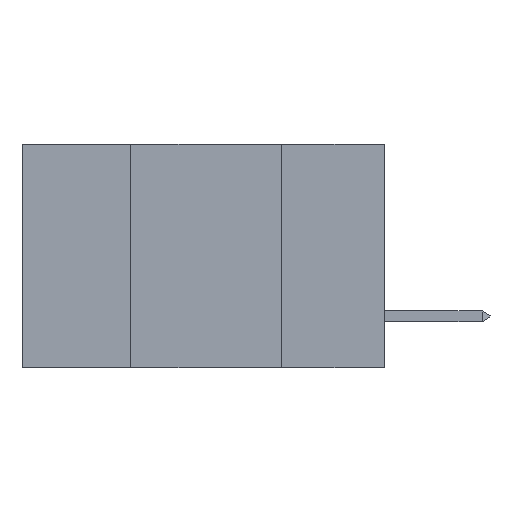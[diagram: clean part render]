
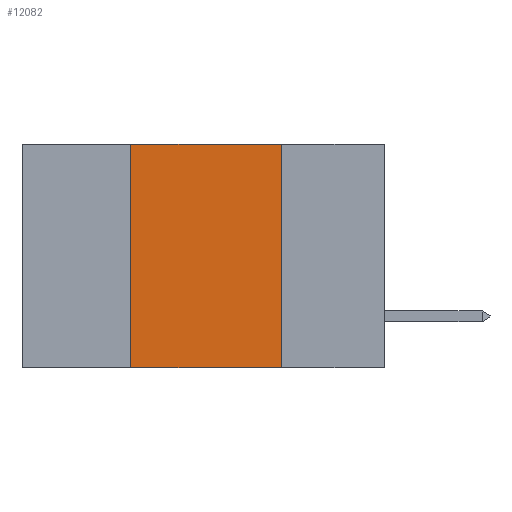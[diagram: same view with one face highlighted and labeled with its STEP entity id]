
A CAD part, left-side view. The second image highlights one B-rep face of the part: STEP entity #12082.
In plain terms, the highlighted planar face has unit normal (-1, 0, 0).
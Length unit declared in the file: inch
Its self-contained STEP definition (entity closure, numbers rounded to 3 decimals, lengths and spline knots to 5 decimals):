
#200 = VECTOR ( 'NONE', #7000, 39.37008 ) ;
#352 = LINE ( 'NONE', #3620, #3742 ) ;
#527 = ORIENTED_EDGE ( 'NONE', *, *, #12980, .T. ) ;
#578 = DIRECTION ( 'NONE',  ( 0., -1., 0. ) ) ;
#1085 = LINE ( 'NONE', #6597, #13701 ) ;
#1118 = CARTESIAN_POINT ( 'NONE',  ( 0., 0.42, 0. ) ) ;
#1951 = EDGE_CURVE ( 'NONE', #12165, #3316, #4775, .T. ) ;
#3173 = DIRECTION ( 'NONE',  ( 1., 0., 0. ) ) ;
#3300 = AXIS2_PLACEMENT_3D ( 'NONE', #7653, #3173, #4312 ) ;
#3316 = VERTEX_POINT ( 'NONE', #6538 ) ;
#3485 = DIRECTION ( 'NONE',  ( 0., -1., 0. ) ) ;
#3620 = CARTESIAN_POINT ( 'NONE',  ( 0., 0.6, -0.37 ) ) ;
#3742 = VECTOR ( 'NONE', #3485, 39.37008 ) ;
#4279 = EDGE_CURVE ( 'NONE', #8274, #12165, #8082, .T. ) ;
#4312 = DIRECTION ( 'NONE',  ( 0., 0., -1. ) ) ;
#4775 = LINE ( 'NONE', #7180, #8708 ) ;
#5139 = ORIENTED_EDGE ( 'NONE', *, *, #4279, .F. ) ;
#6538 = CARTESIAN_POINT ( 'NONE',  ( 0., 0.17, 0. ) ) ;
#6597 = CARTESIAN_POINT ( 'NONE',  ( 0., 0.17, 0. ) ) ;
#6686 = ORIENTED_EDGE ( 'NONE', *, *, #1951, .F. ) ;
#6718 = CARTESIAN_POINT ( 'NONE',  ( 0., 0.42, -0.37 ) ) ;
#7000 = DIRECTION ( 'NONE',  ( 0., 0., 1. ) ) ;
#7180 = CARTESIAN_POINT ( 'NONE',  ( 0., 0.6, 0. ) ) ;
#7653 = CARTESIAN_POINT ( 'NONE',  ( 0., 0.6, 0. ) ) ;
#8082 = LINE ( 'NONE', #1118, #200 ) ;
#8274 = VERTEX_POINT ( 'NONE', #6718 ) ;
#8708 = VECTOR ( 'NONE', #578, 39.37008 ) ;
#8733 = PLANE ( 'NONE',  #3300 ) ;
#10861 = VERTEX_POINT ( 'NONE', #12365 ) ;
#11112 = DIRECTION ( 'NONE',  ( 0., 0., -1. ) ) ;
#11236 = EDGE_CURVE ( 'NONE', #3316, #10861, #1085, .T. ) ;
#11942 = EDGE_LOOP ( 'NONE', ( #14010, #6686, #5139, #527 ) ) ;
#12082 = ADVANCED_FACE ( 'NONE', ( #13106 ), #8733, .F. ) ;
#12165 = VERTEX_POINT ( 'NONE', #13324 ) ;
#12365 = CARTESIAN_POINT ( 'NONE',  ( 0., 0.17, -0.37 ) ) ;
#12980 = EDGE_CURVE ( 'NONE', #8274, #10861, #352, .T. ) ;
#13106 = FACE_OUTER_BOUND ( 'NONE', #11942, .T. ) ;
#13324 = CARTESIAN_POINT ( 'NONE',  ( 0., 0.42, 0. ) ) ;
#13701 = VECTOR ( 'NONE', #11112, 39.37008 ) ;
#14010 = ORIENTED_EDGE ( 'NONE', *, *, #11236, .F. ) ;
